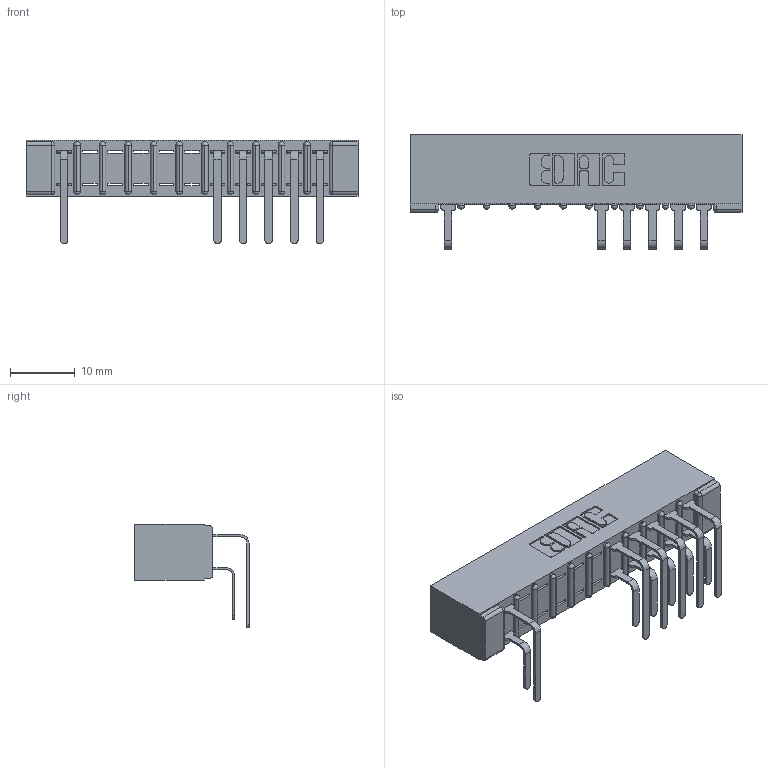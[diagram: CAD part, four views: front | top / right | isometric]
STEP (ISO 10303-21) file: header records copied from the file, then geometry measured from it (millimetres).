
FILE_DESCRIPTION (( 'STEP AP203' ), '1' );
FILE_NAME ('307-011-559-101.STEP', '2018-08-02T21:52:14', ( '' ), ( '' ), 'SwSTEP 2.0', 'SolidWorks 2016', '' );
FILE_SCHEMA (( 'CONFIG_CONTROL_DESIGN' ));
Length unit declared in the file: inch
Products named in the file (4): 307 Part_No Mounting Lugs; 307-290-001_558 559 - 1 (Single); 307-290-001_559 - 2 (Single); 307-011-559-101
Assembly tree (13 placements, depth 2):
  307-011-559-101
    307 Part_No Mounting Lugs
    307-290-001_558 559 - 1 (Single)  x6
    307-290-001_559 - 2 (Single)  x6
Bounding box: 51.46 x 17.69 x 16.08 mm (x, y, z)
Volume: 3524.1 mm3; surface area: 5656.4 mm2
Topology: 13 solids, 13 shells, 822 faces, 2323 edges, 1498 vertices
Faces by surface type: plane 522, cylinder 276, sphere 24
Entity records: 14453 total; most frequent: CARTESIAN_POINT 2415, ORIENTED_EDGE 2398, DIRECTION 2367, EDGE_CURVE 1199, LINE 907, VECTOR 907, VERTEX_POINT 778, AXIS2_PLACEMENT_3D 730
